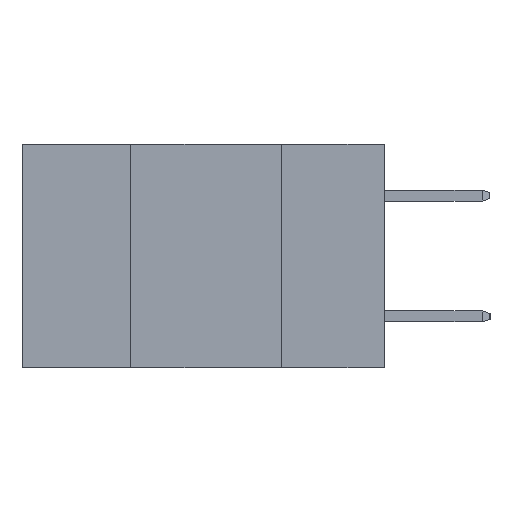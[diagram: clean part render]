
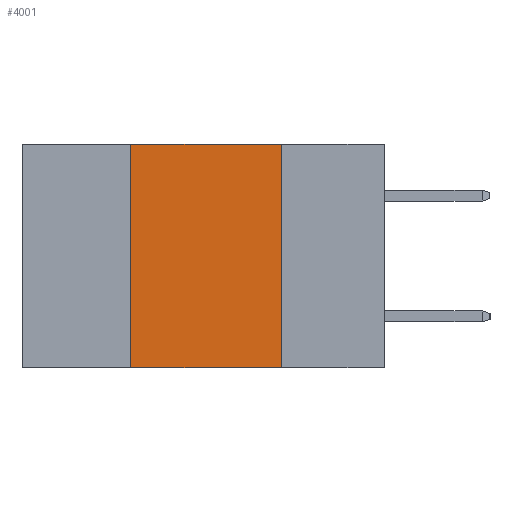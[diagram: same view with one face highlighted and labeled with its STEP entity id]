
A CAD part, left-side view. The second image highlights one B-rep face of the part: STEP entity #4001.
In plain terms, the highlighted planar face has unit normal (-1, 0, 0).
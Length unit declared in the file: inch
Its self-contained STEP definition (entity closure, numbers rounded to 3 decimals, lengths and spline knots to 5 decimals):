
#246 = CARTESIAN_POINT ( 'NONE',  ( 0., 0.17, -0.37 ) ) ;
#371 = CARTESIAN_POINT ( 'NONE',  ( 0., 0.42, -0.37 ) ) ;
#985 = AXIS2_PLACEMENT_3D ( 'NONE', #12326, #12202, #12128 ) ;
#995 = ORIENTED_EDGE ( 'NONE', *, *, #9622, .F. ) ;
#1032 = DIRECTION ( 'NONE',  ( 0., -1., 0. ) ) ;
#1075 = VECTOR ( 'NONE', #7223, 39.37008 ) ;
#1774 = EDGE_LOOP ( 'NONE', ( #9178, #995, #2071, #2602 ) ) ;
#2071 = ORIENTED_EDGE ( 'NONE', *, *, #8216, .F. ) ;
#2253 = EDGE_CURVE ( 'NONE', #7370, #7696, #9436, .T. ) ;
#2602 = ORIENTED_EDGE ( 'NONE', *, *, #7501, .T. ) ;
#2901 = FACE_OUTER_BOUND ( 'NONE', #1774, .T. ) ;
#3573 = DIRECTION ( 'NONE',  ( 0., 0., -1. ) ) ;
#3602 = CARTESIAN_POINT ( 'NONE',  ( 0., 0.17, -0.37 ) ) ;
#3636 = LINE ( 'NONE', #13268, #1075 ) ;
#4001 = ADVANCED_FACE ( 'NONE', ( #2901 ), #12527, .F. ) ;
#4974 = LINE ( 'NONE', #8540, #6480 ) ;
#5166 = CARTESIAN_POINT ( 'NONE',  ( 0., 0.17, 0. ) ) ;
#5965 = LINE ( 'NONE', #10720, #11205 ) ;
#6297 = VECTOR ( 'NONE', #3573, 39.37008 ) ;
#6424 = VERTEX_POINT ( 'NONE', #371 ) ;
#6480 = VECTOR ( 'NONE', #1032, 39.37008 ) ;
#7223 = DIRECTION ( 'NONE',  ( 0., -1., 0. ) ) ;
#7370 = VERTEX_POINT ( 'NONE', #5166 ) ;
#7501 = EDGE_CURVE ( 'NONE', #6424, #7696, #4974, .T. ) ;
#7550 = DIRECTION ( 'NONE',  ( 0., 0., 1. ) ) ;
#7696 = VERTEX_POINT ( 'NONE', #246 ) ;
#8195 = CARTESIAN_POINT ( 'NONE',  ( 0., 0.42, 0. ) ) ;
#8216 = EDGE_CURVE ( 'NONE', #6424, #8536, #5965, .T. ) ;
#8536 = VERTEX_POINT ( 'NONE', #8195 ) ;
#8540 = CARTESIAN_POINT ( 'NONE',  ( 0., 0.6, -0.37 ) ) ;
#9178 = ORIENTED_EDGE ( 'NONE', *, *, #2253, .F. ) ;
#9436 = LINE ( 'NONE', #3602, #6297 ) ;
#9622 = EDGE_CURVE ( 'NONE', #8536, #7370, #3636, .T. ) ;
#10720 = CARTESIAN_POINT ( 'NONE',  ( 0., 0.42, -0.37 ) ) ;
#11205 = VECTOR ( 'NONE', #7550, 39.37008 ) ;
#12128 = DIRECTION ( 'NONE',  ( 0., 0., -1. ) ) ;
#12202 = DIRECTION ( 'NONE',  ( 1., 0., 0. ) ) ;
#12326 = CARTESIAN_POINT ( 'NONE',  ( 0., 0.6, 0. ) ) ;
#12527 = PLANE ( 'NONE',  #985 ) ;
#13268 = CARTESIAN_POINT ( 'NONE',  ( 0., 0.6, 0. ) ) ;
